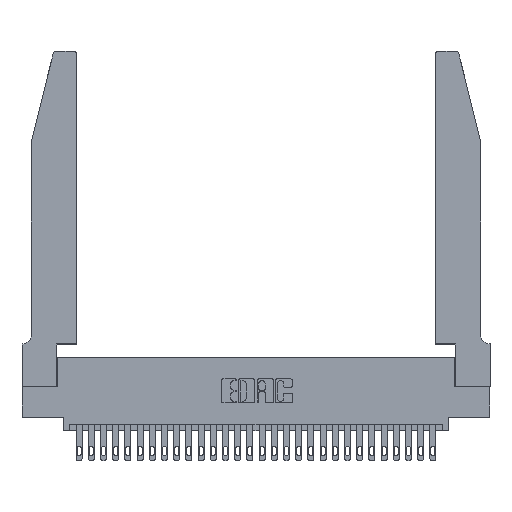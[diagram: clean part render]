
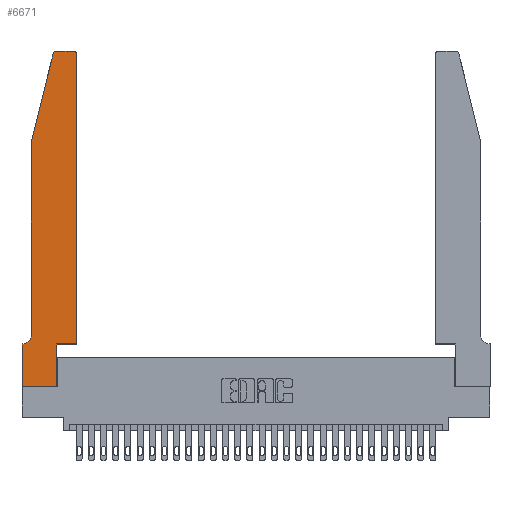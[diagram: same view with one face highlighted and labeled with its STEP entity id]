
A CAD part, top view. The second image highlights one B-rep face of the part: STEP entity #6671.
In plain terms, the highlighted planar face has unit normal (0, 0, 1).
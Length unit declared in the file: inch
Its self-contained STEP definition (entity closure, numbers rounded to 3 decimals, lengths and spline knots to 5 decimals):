
#1 = VECTOR ( 'NONE', #23276, 39.37008 ) ;
#37 = ORIENTED_EDGE ( 'NONE', *, *, #15054, .T. ) ;
#547 = CARTESIAN_POINT ( 'NONE',  ( 0.284, 2.75, 0.37 ) ) ;
#1095 = AXIS2_PLACEMENT_3D ( 'NONE', #20138, #6306, #8606 ) ;
#1464 = CARTESIAN_POINT ( 'NONE',  ( 0., 0., 0.37 ) ) ;
#1897 = VECTOR ( 'NONE', #23966, 39.37008 ) ;
#2140 = ORIENTED_EDGE ( 'NONE', *, *, #26886, .T. ) ;
#2158 = CARTESIAN_POINT ( 'NONE',  ( 0.0755, 0.42, 0.37 ) ) ;
#2246 = CIRCLE ( 'NONE', #1095, 0.07 ) ;
#2877 = DIRECTION ( 'NONE',  ( -1., 0., 0. ) ) ;
#2908 = VECTOR ( 'NONE', #2986, 39.37008 ) ;
#2986 = DIRECTION ( 'NONE',  ( -1., 0., 0. ) ) ;
#3098 = VERTEX_POINT ( 'NONE', #17039 ) ;
#3454 = EDGE_CURVE ( 'NONE', #3098, #28940, #23897, .T. ) ;
#3458 = ORIENTED_EDGE ( 'NONE', *, *, #9740, .T. ) ;
#3975 = ORIENTED_EDGE ( 'NONE', *, *, #16631, .T. ) ;
#4898 = ORIENTED_EDGE ( 'NONE', *, *, #25122, .T. ) ;
#5375 = VECTOR ( 'NONE', #2877, 39.37008 ) ;
#5459 = AXIS2_PLACEMENT_3D ( 'NONE', #25004, #29543, #22569 ) ;
#6306 = DIRECTION ( 'NONE',  ( 0., 0., -1. ) ) ;
#6437 = CARTESIAN_POINT ( 'NONE',  ( 0.4505, 0.35, 0.37 ) ) ;
#6640 = ORIENTED_EDGE ( 'NONE', *, *, #3454, .T. ) ;
#6652 = DIRECTION ( 'NONE',  ( 0., 1., 0. ) ) ;
#6665 = CARTESIAN_POINT ( 'NONE',  ( 0., 0.35, 0.37 ) ) ;
#6671 = ADVANCED_FACE ( 'NONE', ( #17087 ), #22571, .T. ) ;
#7134 = VERTEX_POINT ( 'NONE', #2158 ) ;
#7466 = DIRECTION ( 'NONE',  ( 0., 0., 1. ) ) ;
#7607 = ORIENTED_EDGE ( 'NONE', *, *, #10047, .T. ) ;
#7811 = CARTESIAN_POINT ( 'NONE',  ( 0.0755, 2., 0.37 ) ) ;
#8279 = EDGE_CURVE ( 'NONE', #10107, #3098, #27523, .T. ) ;
#8606 = DIRECTION ( 'NONE',  ( -1., 0., 0. ) ) ;
#9006 = CARTESIAN_POINT ( 'NONE',  ( 0.0055, 0.35, 0.37 ) ) ;
#9687 = DIRECTION ( 'NONE',  ( 1., 0., 0. ) ) ;
#9740 = EDGE_CURVE ( 'NONE', #12171, #19351, #13003, .T. ) ;
#10047 = EDGE_CURVE ( 'NONE', #25450, #7134, #28165, .T. ) ;
#10054 = CIRCLE ( 'NONE', #5459, 0.03 ) ;
#10107 = VERTEX_POINT ( 'NONE', #1464 ) ;
#10116 = VECTOR ( 'NONE', #23105, 39.37008 ) ;
#10217 = EDGE_LOOP ( 'NONE', ( #3458, #23374, #14303, #7607, #4898, #2140, #14862, #14640, #6640, #37, #25014, #3975 ) ) ;
#10459 = DIRECTION ( 'NONE',  ( 0., -1., 0. ) ) ;
#10905 = VECTOR ( 'NONE', #6652, 39.37008 ) ;
#11331 = CARTESIAN_POINT ( 'NONE',  ( 0.4505, 0.35, 0.37 ) ) ;
#11526 = EDGE_CURVE ( 'NONE', #19351, #26456, #26999, .T. ) ;
#11775 = AXIS2_PLACEMENT_3D ( 'NONE', #12156, #7466, #9687 ) ;
#12087 = LINE ( 'NONE', #7811, #1897 ) ;
#12156 = CARTESIAN_POINT ( 'NONE',  ( 0.284, 2.72, 0.37 ) ) ;
#12171 = VERTEX_POINT ( 'NONE', #23563 ) ;
#13003 = LINE ( 'NONE', #14615, #5375 ) ;
#13043 = AXIS2_PLACEMENT_3D ( 'NONE', #29449, #13489, #15781 ) ;
#13489 = DIRECTION ( 'NONE',  ( 0., 0., 1. ) ) ;
#14303 = ORIENTED_EDGE ( 'NONE', *, *, #29100, .T. ) ;
#14378 = VECTOR ( 'NONE', #20098, 39.37008 ) ;
#14457 = VECTOR ( 'NONE', #10459, 39.37008 ) ;
#14585 = CARTESIAN_POINT ( 'NONE',  ( 0., 0., 0.37 ) ) ;
#14615 = CARTESIAN_POINT ( 'NONE',  ( 0.2605, 2.75, 0.37 ) ) ;
#14625 = CARTESIAN_POINT ( 'NONE',  ( 0.0755, 2., 0.37 ) ) ;
#14640 = ORIENTED_EDGE ( 'NONE', *, *, #8279, .T. ) ;
#14732 = EDGE_CURVE ( 'NONE', #23791, #10107, #20624, .T. ) ;
#14862 = ORIENTED_EDGE ( 'NONE', *, *, #14732, .T. ) ;
#15054 = EDGE_CURVE ( 'NONE', #28940, #17808, #21349, .T. ) ;
#15696 = EDGE_CURVE ( 'NONE', #17808, #28094, #24593, .T. ) ;
#15781 = DIRECTION ( 'NONE',  ( 1., 0., 0. ) ) ;
#15980 = DIRECTION ( 'NONE',  ( 1., 0., 0. ) ) ;
#16631 = EDGE_CURVE ( 'NONE', #28094, #12171, #10054, .T. ) ;
#16914 = CARTESIAN_POINT ( 'NONE',  ( 0., 0., 0.37 ) ) ;
#17039 = CARTESIAN_POINT ( 'NONE',  ( 0.2865, 0., 0.37 ) ) ;
#17087 = FACE_OUTER_BOUND ( 'NONE', #10217, .T. ) ;
#17808 = VERTEX_POINT ( 'NONE', #6437 ) ;
#19298 = CARTESIAN_POINT ( 'NONE',  ( 0.0755, 0.35, 0.37 ) ) ;
#19351 = VERTEX_POINT ( 'NONE', #547 ) ;
#20098 = DIRECTION ( 'NONE',  ( 0., -1., 0. ) ) ;
#20138 = CARTESIAN_POINT ( 'NONE',  ( 0.0055, 0.42, 0.37 ) ) ;
#20624 = LINE ( 'NONE', #16914, #14457 ) ;
#21349 = LINE ( 'NONE', #27501, #22053 ) ;
#21382 = LINE ( 'NONE', #19298, #2908 ) ;
#22053 = VECTOR ( 'NONE', #15980, 39.37008 ) ;
#22336 = CARTESIAN_POINT ( 'NONE',  ( 0.25487, 2.72718, 0.37 ) ) ;
#22569 = DIRECTION ( 'NONE',  ( 1., 0., 0. ) ) ;
#22571 = PLANE ( 'NONE',  #13043 ) ;
#23105 = DIRECTION ( 'NONE',  ( 0., 1., 0. ) ) ;
#23276 = DIRECTION ( 'NONE',  ( 1., 0., 0. ) ) ;
#23374 = ORIENTED_EDGE ( 'NONE', *, *, #11526, .T. ) ;
#23563 = CARTESIAN_POINT ( 'NONE',  ( 0.4205, 2.75, 0.37 ) ) ;
#23791 = VERTEX_POINT ( 'NONE', #6665 ) ;
#23897 = LINE ( 'NONE', #27455, #10905 ) ;
#23966 = DIRECTION ( 'NONE',  ( -0.239, -0.971, 0. ) ) ;
#24593 = LINE ( 'NONE', #11331, #10116 ) ;
#25004 = CARTESIAN_POINT ( 'NONE',  ( 0.4205, 2.72, 0.37 ) ) ;
#25014 = ORIENTED_EDGE ( 'NONE', *, *, #15696, .T. ) ;
#25122 = EDGE_CURVE ( 'NONE', #7134, #29591, #2246, .T. ) ;
#25450 = VERTEX_POINT ( 'NONE', #14625 ) ;
#26456 = VERTEX_POINT ( 'NONE', #22336 ) ;
#26886 = EDGE_CURVE ( 'NONE', #29591, #23791, #21382, .T. ) ;
#26999 = CIRCLE ( 'NONE', #11775, 0.03 ) ;
#27356 = CARTESIAN_POINT ( 'NONE',  ( 0.2865, 0.35, 0.37 ) ) ;
#27455 = CARTESIAN_POINT ( 'NONE',  ( 0.2865, 0.35, 0.37 ) ) ;
#27501 = CARTESIAN_POINT ( 'NONE',  ( 0.4505, 0.35, 0.37 ) ) ;
#27523 = LINE ( 'NONE', #14585, #1 ) ;
#28094 = VERTEX_POINT ( 'NONE', #28817 ) ;
#28165 = LINE ( 'NONE', #29177, #14378 ) ;
#28817 = CARTESIAN_POINT ( 'NONE',  ( 0.4505, 2.72, 0.37 ) ) ;
#28940 = VERTEX_POINT ( 'NONE', #27356 ) ;
#29100 = EDGE_CURVE ( 'NONE', #26456, #25450, #12087, .T. ) ;
#29177 = CARTESIAN_POINT ( 'NONE',  ( 0.0755, 2., 0.37 ) ) ;
#29449 = CARTESIAN_POINT ( 'NONE',  ( 0., 0.35, 0.37 ) ) ;
#29543 = DIRECTION ( 'NONE',  ( 0., 0., 1. ) ) ;
#29591 = VERTEX_POINT ( 'NONE', #9006 ) ;
